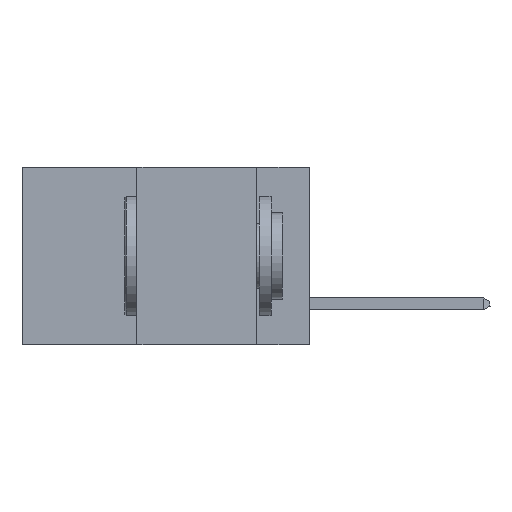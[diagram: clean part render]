
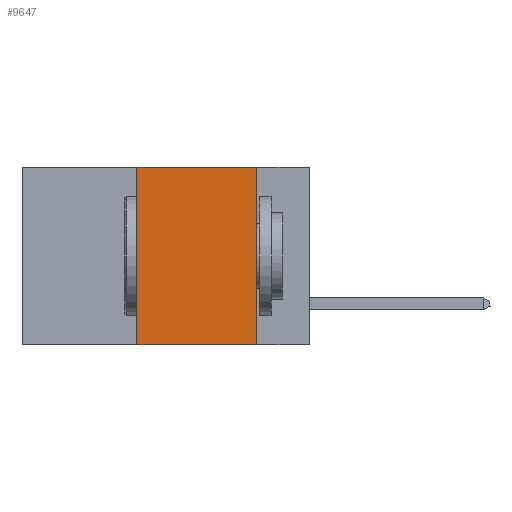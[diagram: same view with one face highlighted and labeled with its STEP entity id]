
A CAD part, left-side view. The second image highlights one B-rep face of the part: STEP entity #9647.
In plain terms, the highlighted planar face has unit normal (-1, 0, 0).
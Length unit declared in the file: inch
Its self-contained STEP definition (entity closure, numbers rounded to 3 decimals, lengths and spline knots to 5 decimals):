
#996 = VECTOR ( 'NONE', #1360, 39.37008 ) ;
#1360 = DIRECTION ( 'NONE',  ( 0., -1., 0. ) ) ;
#1908 = LINE ( 'NONE', #12444, #20035 ) ;
#1958 = EDGE_CURVE ( 'NONE', #10882, #1982, #8725, .T. ) ;
#1982 = VERTEX_POINT ( 'NONE', #3673 ) ;
#2569 = AXIS2_PLACEMENT_3D ( 'NONE', #15395, #7577, #9291 ) ;
#3210 = CARTESIAN_POINT ( 'NONE',  ( 0., 0.11, 0. ) ) ;
#3673 = CARTESIAN_POINT ( 'NONE',  ( 0., 0.36, 0. ) ) ;
#3930 = DIRECTION ( 'NONE',  ( 0., 0., 1. ) ) ;
#3999 = EDGE_CURVE ( 'NONE', #1982, #9084, #9399, .T. ) ;
#4387 = EDGE_LOOP ( 'NONE', ( #15568, #4409, #5071, #18280 ) ) ;
#4409 = ORIENTED_EDGE ( 'NONE', *, *, #3999, .F. ) ;
#5071 = ORIENTED_EDGE ( 'NONE', *, *, #1958, .F. ) ;
#6148 = LINE ( 'NONE', #3210, #6610 ) ;
#6496 = CARTESIAN_POINT ( 'NONE',  ( 0., 0.11, -0.37 ) ) ;
#6610 = VECTOR ( 'NONE', #14335, 39.37008 ) ;
#6795 = CARTESIAN_POINT ( 'NONE',  ( 0., 0.36, 0. ) ) ;
#7019 = CARTESIAN_POINT ( 'NONE',  ( 0., 0.6, 0. ) ) ;
#7577 = DIRECTION ( 'NONE',  ( 1., 0., 0. ) ) ;
#8207 = EDGE_CURVE ( 'NONE', #9084, #16359, #6148, .T. ) ;
#8704 = CARTESIAN_POINT ( 'NONE',  ( 0., 0.36, -0.37 ) ) ;
#8725 = LINE ( 'NONE', #6795, #16519 ) ;
#8751 = EDGE_CURVE ( 'NONE', #10882, #16359, #1908, .T. ) ;
#8813 = PLANE ( 'NONE',  #2569 ) ;
#9084 = VERTEX_POINT ( 'NONE', #9153 ) ;
#9153 = CARTESIAN_POINT ( 'NONE',  ( 0., 0.11, 0. ) ) ;
#9291 = DIRECTION ( 'NONE',  ( 0., 0., -1. ) ) ;
#9399 = LINE ( 'NONE', #7019, #996 ) ;
#9647 = ADVANCED_FACE ( 'NONE', ( #19286 ), #8813, .F. ) ;
#10882 = VERTEX_POINT ( 'NONE', #8704 ) ;
#12444 = CARTESIAN_POINT ( 'NONE',  ( 0., 0.6, -0.37 ) ) ;
#14335 = DIRECTION ( 'NONE',  ( 0., 0., -1. ) ) ;
#15395 = CARTESIAN_POINT ( 'NONE',  ( 0., 0.6, 0. ) ) ;
#15568 = ORIENTED_EDGE ( 'NONE', *, *, #8207, .F. ) ;
#16359 = VERTEX_POINT ( 'NONE', #6496 ) ;
#16519 = VECTOR ( 'NONE', #3930, 39.37008 ) ;
#17294 = DIRECTION ( 'NONE',  ( 0., -1., 0. ) ) ;
#18280 = ORIENTED_EDGE ( 'NONE', *, *, #8751, .T. ) ;
#19286 = FACE_OUTER_BOUND ( 'NONE', #4387, .T. ) ;
#20035 = VECTOR ( 'NONE', #17294, 39.37008 ) ;
